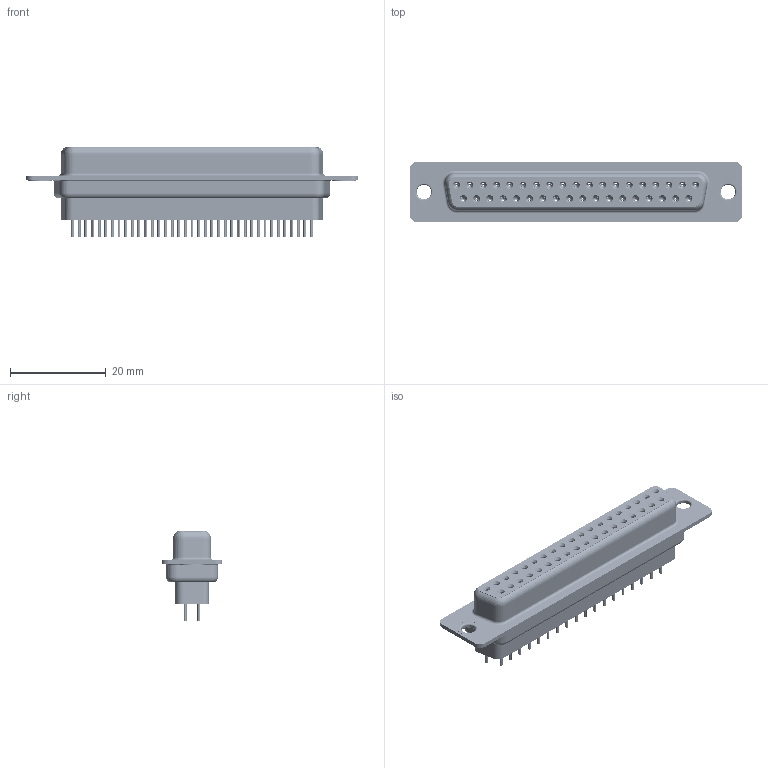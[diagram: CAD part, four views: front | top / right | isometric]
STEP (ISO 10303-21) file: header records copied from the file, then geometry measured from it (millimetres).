
FILE_DESCRIPTION (( 'STEP AP203' ), '1' );
FILE_NAME ('628-037-228-241.STEP', '2020-07-21T00:39:59', ( '' ), ( '' ), 'SwSTEP 2.0', 'SolidWorks 2020', '' );
FILE_SCHEMA (( 'CONFIG_CONTROL_DESIGN' ));
Length unit declared in the file: millimetre
Products named in the file (7): 628 Shell Front_37 Contacts; 628 Housing_37 FF; 628-037-228-241; 628 Contact Row 2_28L; 628 Thru Hole Rivet; 628 Shell Rear_37 Contacts; 628 Contact Row 1_28L
Assembly tree (42 placements, depth 2):
  628-037-228-241
    628 Housing_37 FF
    628 Shell Front_37 Contacts
    628 Shell Rear_37 Contacts
    628 Contact Row 1_28L  x19
    628 Contact Row 2_28L  x18
    628 Thru Hole Rivet  x2
Bounding box: 69.3 x 12.6 x 18.8 mm (x, y, z)
Volume: 6142.4 mm3; surface area: 13831.6 mm2
Topology: 42 solids, 42 shells, 4952 faces, 12591 edges, 7808 vertices
Faces by surface type: cylinder 1342, plane 1214, torus 1027, bspline 740, cone 629
Entity records: 30919 total; most frequent: CARTESIAN_POINT 7095, DIRECTION 4985, ORIENTED_EDGE 4362, EDGE_CURVE 2181, AXIS2_PLACEMENT_3D 2104, VERTEX_POINT 1375, CIRCLE 1161, EDGE_LOOP 1146
